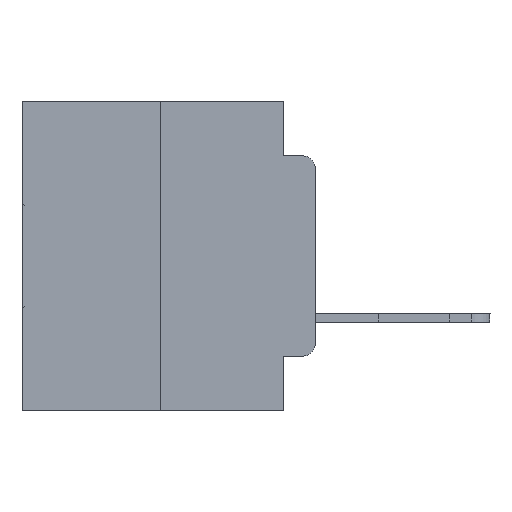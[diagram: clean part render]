
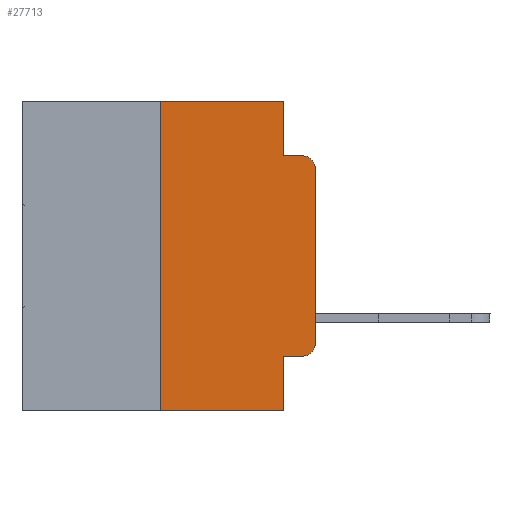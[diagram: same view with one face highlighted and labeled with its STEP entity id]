
A CAD part, left-side view. The second image highlights one B-rep face of the part: STEP entity #27713.
In plain terms, the highlighted planar face has unit normal (-1, 0, 0).
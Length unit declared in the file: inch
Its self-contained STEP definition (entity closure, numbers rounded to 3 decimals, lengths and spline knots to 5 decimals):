
#111 = CARTESIAN_POINT ( 'NONE',  ( 0., 0., -0.1085 ) ) ;
#369 = CARTESIAN_POINT ( 'NONE',  ( 0., 0.473, 0. ) ) ;
#677 = DIRECTION ( 'NONE',  ( 0., 0., -1. ) ) ;
#1460 = LINE ( 'NONE', #6560, #6236 ) ;
#1719 = CARTESIAN_POINT ( 'NONE',  ( 0., 0.051, -0.4115 ) ) ;
#2174 = DIRECTION ( 'NONE',  ( 0., 0., -1. ) ) ;
#2758 = EDGE_CURVE ( 'NONE', #13812, #10153, #25540, .T. ) ;
#4308 = CIRCLE ( 'NONE', #25515, 0.02 ) ;
#4551 = DIRECTION ( 'NONE',  ( 0., -1., 0. ) ) ;
#4809 = AXIS2_PLACEMENT_3D ( 'NONE', #17129, #29012, #26524 ) ;
#4988 = VECTOR ( 'NONE', #30495, 39.37008 ) ;
#5301 = CIRCLE ( 'NONE', #4809, 0.02 ) ;
#5325 = ORIENTED_EDGE ( 'NONE', *, *, #22782, .T. ) ;
#5485 = VERTEX_POINT ( 'NONE', #11689 ) ;
#6168 = DIRECTION ( 'NONE',  ( 0., 0., 1. ) ) ;
#6184 = ORIENTED_EDGE ( 'NONE', *, *, #13692, .T. ) ;
#6236 = VECTOR ( 'NONE', #29759, 39.37008 ) ;
#6511 = LINE ( 'NONE', #30160, #28314 ) ;
#6560 = CARTESIAN_POINT ( 'NONE',  ( 0., 0.25, 0. ) ) ;
#6787 = EDGE_CURVE ( 'NONE', #13812, #15687, #1460, .T. ) ;
#8047 = CARTESIAN_POINT ( 'NONE',  ( 0., 0.25, -0.5 ) ) ;
#8183 = LINE ( 'NONE', #18211, #20067 ) ;
#8237 = EDGE_CURVE ( 'NONE', #19992, #17706, #4308, .T. ) ;
#9441 = EDGE_CURVE ( 'NONE', #10563, #10153, #21865, .T. ) ;
#9507 = EDGE_CURVE ( 'NONE', #15687, #5485, #23707, .T. ) ;
#9810 = ORIENTED_EDGE ( 'NONE', *, *, #9507, .F. ) ;
#9823 = DIRECTION ( 'NONE',  ( 0., -1., 0. ) ) ;
#10153 = VERTEX_POINT ( 'NONE', #29989 ) ;
#10253 = VECTOR ( 'NONE', #9823, 39.37008 ) ;
#10563 = VERTEX_POINT ( 'NONE', #1719 ) ;
#11102 = VECTOR ( 'NONE', #4551, 39.37008 ) ;
#11640 = CARTESIAN_POINT ( 'NONE',  ( 0., 0.051, -0.4115 ) ) ;
#11689 = CARTESIAN_POINT ( 'NONE',  ( 0., 0.051, 0. ) ) ;
#12827 = CARTESIAN_POINT ( 'NONE',  ( 0., 0.051, -0.0885 ) ) ;
#12938 = CARTESIAN_POINT ( 'NONE',  ( 0., 0.25, 0. ) ) ;
#13692 = EDGE_CURVE ( 'NONE', #10563, #19992, #30187, .T. ) ;
#13812 = VERTEX_POINT ( 'NONE', #8047 ) ;
#13983 = ORIENTED_EDGE ( 'NONE', *, *, #19805, .F. ) ;
#14148 = FACE_OUTER_BOUND ( 'NONE', #16653, .T. ) ;
#14759 = CARTESIAN_POINT ( 'NONE',  ( 0., 0.051, 0. ) ) ;
#14761 = CARTESIAN_POINT ( 'NONE',  ( 0., 0.473, 0. ) ) ;
#15476 = VERTEX_POINT ( 'NONE', #111 ) ;
#15687 = VERTEX_POINT ( 'NONE', #12938 ) ;
#15695 = VERTEX_POINT ( 'NONE', #26984 ) ;
#16653 = EDGE_LOOP ( 'NONE', ( #5325, #20296, #23957, #13983, #9810, #23537, #30060, #22972, #6184, #29023 ) ) ;
#17117 = VECTOR ( 'NONE', #22243, 39.37008 ) ;
#17129 = CARTESIAN_POINT ( 'NONE',  ( 0., 0.02, -0.1085 ) ) ;
#17706 = VERTEX_POINT ( 'NONE', #21529 ) ;
#17785 = CARTESIAN_POINT ( 'NONE',  ( 0., 0.02, -0.4115 ) ) ;
#18211 = CARTESIAN_POINT ( 'NONE',  ( 0., 0., 0. ) ) ;
#18780 = DIRECTION ( 'NONE',  ( 0., 0., -1. ) ) ;
#19088 = DIRECTION ( 'NONE',  ( -1., 0., 0. ) ) ;
#19805 = EDGE_CURVE ( 'NONE', #5485, #28924, #6511, .T. ) ;
#19992 = VERTEX_POINT ( 'NONE', #17785 ) ;
#20067 = VECTOR ( 'NONE', #6168, 39.37008 ) ;
#20296 = ORIENTED_EDGE ( 'NONE', *, *, #23051, .T. ) ;
#21529 = CARTESIAN_POINT ( 'NONE',  ( 0., 0., -0.3915 ) ) ;
#21865 = LINE ( 'NONE', #14759, #26031 ) ;
#22243 = DIRECTION ( 'NONE',  ( 0., -1., 0. ) ) ;
#22782 = EDGE_CURVE ( 'NONE', #17706, #15476, #8183, .T. ) ;
#22972 = ORIENTED_EDGE ( 'NONE', *, *, #9441, .F. ) ;
#23051 = EDGE_CURVE ( 'NONE', #15476, #15695, #5301, .T. ) ;
#23537 = ORIENTED_EDGE ( 'NONE', *, *, #6787, .F. ) ;
#23707 = LINE ( 'NONE', #369, #10253 ) ;
#23861 = DIRECTION ( 'NONE',  ( 1., 0., 0. ) ) ;
#23932 = EDGE_CURVE ( 'NONE', #28924, #15695, #24551, .T. ) ;
#23957 = ORIENTED_EDGE ( 'NONE', *, *, #23932, .F. ) ;
#24551 = LINE ( 'NONE', #12827, #17117 ) ;
#24658 = AXIS2_PLACEMENT_3D ( 'NONE', #14761, #23861, #28970 ) ;
#25515 = AXIS2_PLACEMENT_3D ( 'NONE', #26178, #19088, #18780 ) ;
#25540 = LINE ( 'NONE', #25697, #11102 ) ;
#25697 = CARTESIAN_POINT ( 'NONE',  ( 0., 0.473, -0.5 ) ) ;
#26031 = VECTOR ( 'NONE', #677, 39.37008 ) ;
#26178 = CARTESIAN_POINT ( 'NONE',  ( 0., 0.02, -0.3915 ) ) ;
#26524 = DIRECTION ( 'NONE',  ( 0., 0., -1. ) ) ;
#26648 = CARTESIAN_POINT ( 'NONE',  ( 0., 0.051, -0.0885 ) ) ;
#26984 = CARTESIAN_POINT ( 'NONE',  ( 0., 0.02, -0.0885 ) ) ;
#27713 = ADVANCED_FACE ( 'NONE', ( #14148 ), #28512, .F. ) ;
#28314 = VECTOR ( 'NONE', #2174, 39.37008 ) ;
#28512 = PLANE ( 'NONE',  #24658 ) ;
#28924 = VERTEX_POINT ( 'NONE', #26648 ) ;
#28970 = DIRECTION ( 'NONE',  ( 0., 0., -1. ) ) ;
#29012 = DIRECTION ( 'NONE',  ( -1., 0., 0. ) ) ;
#29023 = ORIENTED_EDGE ( 'NONE', *, *, #8237, .T. ) ;
#29759 = DIRECTION ( 'NONE',  ( 0., 0., 1. ) ) ;
#29989 = CARTESIAN_POINT ( 'NONE',  ( 0., 0.051, -0.5 ) ) ;
#30060 = ORIENTED_EDGE ( 'NONE', *, *, #2758, .T. ) ;
#30160 = CARTESIAN_POINT ( 'NONE',  ( 0., 0.051, 0. ) ) ;
#30187 = LINE ( 'NONE', #11640, #4988 ) ;
#30495 = DIRECTION ( 'NONE',  ( 0., -1., 0. ) ) ;
